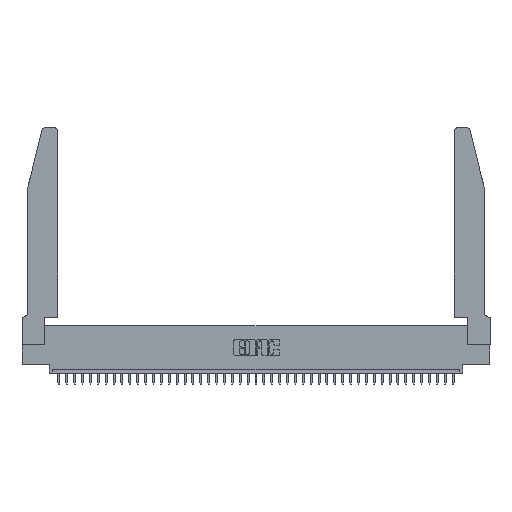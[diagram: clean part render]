
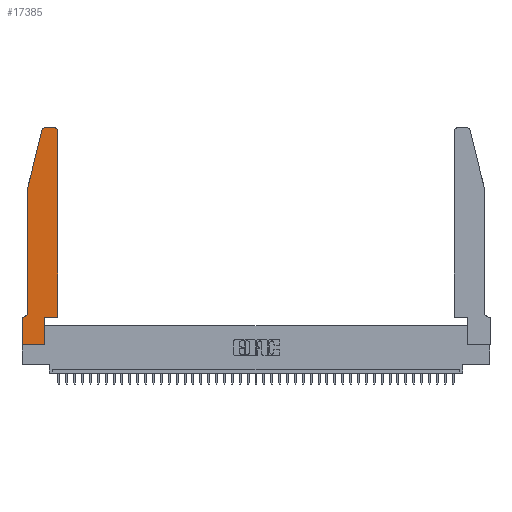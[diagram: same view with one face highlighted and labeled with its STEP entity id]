
A CAD part, top view. The second image highlights one B-rep face of the part: STEP entity #17385.
In plain terms, the highlighted planar face has unit normal (0, 0, 1).
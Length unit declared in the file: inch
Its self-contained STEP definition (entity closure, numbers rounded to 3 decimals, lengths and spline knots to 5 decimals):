
#886 = ORIENTED_EDGE ( 'NONE', *, *, #33752, .T. ) ;
#1189 = CARTESIAN_POINT ( 'NONE',  ( 0., 0.35, 0.37 ) ) ;
#1300 = VERTEX_POINT ( 'NONE', #12497 ) ;
#1903 = AXIS2_PLACEMENT_3D ( 'NONE', #33778, #28754, #16655 ) ;
#2363 = CARTESIAN_POINT ( 'NONE',  ( 0.0755, 0.42, 0.37 ) ) ;
#3239 = LINE ( 'NONE', #35025, #6347 ) ;
#3327 = VECTOR ( 'NONE', #10362, 39.37008 ) ;
#4144 = EDGE_LOOP ( 'NONE', ( #27948, #886, #27463, #6502, #39175, #15847, #22518, #16967, #21735, #23701, #37034, #6998 ) ) ;
#4234 = DIRECTION ( 'NONE',  ( 0., 0., 1. ) ) ;
#4653 = EDGE_CURVE ( 'NONE', #6295, #8956, #20450, .T. ) ;
#5213 = VECTOR ( 'NONE', #21820, 39.37008 ) ;
#5269 = DIRECTION ( 'NONE',  ( 0., 1., 0. ) ) ;
#5425 = CARTESIAN_POINT ( 'NONE',  ( 0.0755, 2., 0.37 ) ) ;
#6295 = VERTEX_POINT ( 'NONE', #31590 ) ;
#6347 = VECTOR ( 'NONE', #6990, 39.37008 ) ;
#6502 = ORIENTED_EDGE ( 'NONE', *, *, #4653, .T. ) ;
#6990 = DIRECTION ( 'NONE',  ( 0., -1., 0. ) ) ;
#6998 = ORIENTED_EDGE ( 'NONE', *, *, #23781, .T. ) ;
#7196 = CARTESIAN_POINT ( 'NONE',  ( 0.0755, 2., 0.37 ) ) ;
#7483 = VERTEX_POINT ( 'NONE', #38653 ) ;
#8956 = VERTEX_POINT ( 'NONE', #2363 ) ;
#9925 = VERTEX_POINT ( 'NONE', #34932 ) ;
#9992 = VERTEX_POINT ( 'NONE', #1189 ) ;
#10031 = AXIS2_PLACEMENT_3D ( 'NONE', #14237, #14657, #11582 ) ;
#10362 = DIRECTION ( 'NONE',  ( 0., 1., 0. ) ) ;
#10498 = DIRECTION ( 'NONE',  ( 1., 0., 0. ) ) ;
#11582 = DIRECTION ( 'NONE',  ( 1., 0., 0. ) ) ;
#12497 = CARTESIAN_POINT ( 'NONE',  ( 0.2865, 0., 0.37 ) ) ;
#12509 = EDGE_CURVE ( 'NONE', #9992, #38305, #3239, .T. ) ;
#12897 = CARTESIAN_POINT ( 'NONE',  ( 0.25487, 2.72718, 0.37 ) ) ;
#13039 = CARTESIAN_POINT ( 'NONE',  ( 0.4505, 2.72, 0.37 ) ) ;
#14237 = CARTESIAN_POINT ( 'NONE',  ( 0., 0.35, 0.37 ) ) ;
#14657 = DIRECTION ( 'NONE',  ( 0., 0., 1. ) ) ;
#14684 = CARTESIAN_POINT ( 'NONE',  ( 0.2605, 2.75, 0.37 ) ) ;
#15847 = ORIENTED_EDGE ( 'NONE', *, *, #28110, .T. ) ;
#16337 = DIRECTION ( 'NONE',  ( 1., 0., 0. ) ) ;
#16551 = CARTESIAN_POINT ( 'NONE',  ( 0.2865, 0.35, 0.37 ) ) ;
#16655 = DIRECTION ( 'NONE',  ( -1., 0., 0. ) ) ;
#16967 = ORIENTED_EDGE ( 'NONE', *, *, #24372, .T. ) ;
#16978 = LINE ( 'NONE', #27880, #18086 ) ;
#17197 = VERTEX_POINT ( 'NONE', #17507 ) ;
#17385 = ADVANCED_FACE ( 'NONE', ( #37191 ), #39342, .T. ) ;
#17389 = VERTEX_POINT ( 'NONE', #38580 ) ;
#17492 = VECTOR ( 'NONE', #22443, 39.37008 ) ;
#17507 = CARTESIAN_POINT ( 'NONE',  ( 0.2865, 0.35, 0.37 ) ) ;
#17993 = VECTOR ( 'NONE', #5269, 39.37008 ) ;
#18086 = VECTOR ( 'NONE', #32997, 39.37008 ) ;
#18588 = EDGE_CURVE ( 'NONE', #31051, #6295, #37106, .T. ) ;
#19074 = EDGE_CURVE ( 'NONE', #8956, #7483, #39080, .T. ) ;
#20450 = LINE ( 'NONE', #5425, #28613 ) ;
#21735 = ORIENTED_EDGE ( 'NONE', *, *, #32597, .T. ) ;
#21820 = DIRECTION ( 'NONE',  ( 1., 0., 0. ) ) ;
#21932 = CARTESIAN_POINT ( 'NONE',  ( 0., 0., 0.37 ) ) ;
#22117 = EDGE_CURVE ( 'NONE', #17197, #9925, #16978, .T. ) ;
#22443 = DIRECTION ( 'NONE',  ( -1., 0., 0. ) ) ;
#22518 = ORIENTED_EDGE ( 'NONE', *, *, #12509, .T. ) ;
#22605 = DIRECTION ( 'NONE',  ( 0., 0., 1. ) ) ;
#22647 = EDGE_CURVE ( 'NONE', #24750, #17389, #24618, .T. ) ;
#22897 = EDGE_CURVE ( 'NONE', #9925, #30875, #31696, .T. ) ;
#22966 = CARTESIAN_POINT ( 'NONE',  ( 0.284, 2.72, 0.37 ) ) ;
#23701 = ORIENTED_EDGE ( 'NONE', *, *, #22117, .T. ) ;
#23781 = EDGE_CURVE ( 'NONE', #30875, #24750, #28051, .T. ) ;
#24372 = EDGE_CURVE ( 'NONE', #38305, #1300, #34615, .T. ) ;
#24618 = LINE ( 'NONE', #14684, #17492 ) ;
#24750 = VERTEX_POINT ( 'NONE', #39697 ) ;
#27463 = ORIENTED_EDGE ( 'NONE', *, *, #18588, .T. ) ;
#27880 = CARTESIAN_POINT ( 'NONE',  ( 0.4505, 0.35, 0.37 ) ) ;
#27948 = ORIENTED_EDGE ( 'NONE', *, *, #22647, .T. ) ;
#28051 = CIRCLE ( 'NONE', #35972, 0.03 ) ;
#28110 = EDGE_CURVE ( 'NONE', #7483, #9992, #32620, .T. ) ;
#28322 = DIRECTION ( 'NONE',  ( 0., -1., 0. ) ) ;
#28613 = VECTOR ( 'NONE', #28322, 39.37008 ) ;
#28754 = DIRECTION ( 'NONE',  ( 0., 0., -1. ) ) ;
#30074 = VECTOR ( 'NONE', #36333, 39.37008 ) ;
#30875 = VERTEX_POINT ( 'NONE', #13039 ) ;
#30946 = VECTOR ( 'NONE', #33534, 39.37008 ) ;
#31051 = VERTEX_POINT ( 'NONE', #12897 ) ;
#31304 = CARTESIAN_POINT ( 'NONE',  ( 0.4505, 0.35, 0.37 ) ) ;
#31590 = CARTESIAN_POINT ( 'NONE',  ( 0.0755, 2., 0.37 ) ) ;
#31696 = LINE ( 'NONE', #31304, #17993 ) ;
#32573 = CARTESIAN_POINT ( 'NONE',  ( 0.4205, 2.72, 0.37 ) ) ;
#32597 = EDGE_CURVE ( 'NONE', #1300, #17197, #37362, .T. ) ;
#32620 = LINE ( 'NONE', #39765, #30074 ) ;
#32997 = DIRECTION ( 'NONE',  ( 1., 0., 0. ) ) ;
#33534 = DIRECTION ( 'NONE',  ( -0.239, -0.971, 0. ) ) ;
#33752 = EDGE_CURVE ( 'NONE', #17389, #31051, #39289, .T. ) ;
#33778 = CARTESIAN_POINT ( 'NONE',  ( 0.0055, 0.42, 0.37 ) ) ;
#34434 = CARTESIAN_POINT ( 'NONE',  ( 0., 0., 0.37 ) ) ;
#34615 = LINE ( 'NONE', #34434, #5213 ) ;
#34932 = CARTESIAN_POINT ( 'NONE',  ( 0.4505, 0.35, 0.37 ) ) ;
#35025 = CARTESIAN_POINT ( 'NONE',  ( 0., 0., 0.37 ) ) ;
#35695 = AXIS2_PLACEMENT_3D ( 'NONE', #22966, #22605, #16337 ) ;
#35972 = AXIS2_PLACEMENT_3D ( 'NONE', #32573, #4234, #10498 ) ;
#36333 = DIRECTION ( 'NONE',  ( -1., 0., 0. ) ) ;
#37034 = ORIENTED_EDGE ( 'NONE', *, *, #22897, .T. ) ;
#37106 = LINE ( 'NONE', #7196, #30946 ) ;
#37191 = FACE_OUTER_BOUND ( 'NONE', #4144, .T. ) ;
#37362 = LINE ( 'NONE', #16551, #3327 ) ;
#38305 = VERTEX_POINT ( 'NONE', #21932 ) ;
#38580 = CARTESIAN_POINT ( 'NONE',  ( 0.284, 2.75, 0.37 ) ) ;
#38653 = CARTESIAN_POINT ( 'NONE',  ( 0.0055, 0.35, 0.37 ) ) ;
#39080 = CIRCLE ( 'NONE', #1903, 0.07 ) ;
#39175 = ORIENTED_EDGE ( 'NONE', *, *, #19074, .T. ) ;
#39289 = CIRCLE ( 'NONE', #35695, 0.03 ) ;
#39342 = PLANE ( 'NONE',  #10031 ) ;
#39697 = CARTESIAN_POINT ( 'NONE',  ( 0.4205, 2.75, 0.37 ) ) ;
#39765 = CARTESIAN_POINT ( 'NONE',  ( 0.0755, 0.35, 0.37 ) ) ;
